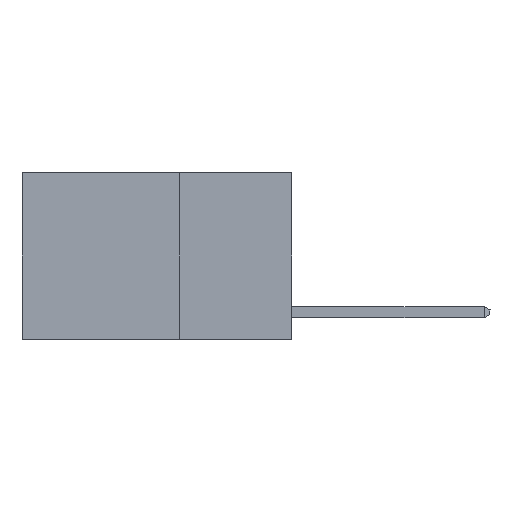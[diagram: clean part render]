
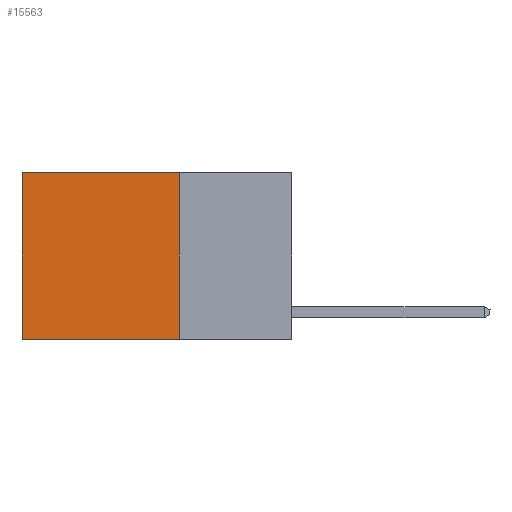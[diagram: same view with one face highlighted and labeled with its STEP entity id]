
A CAD part, left-side view. The second image highlights one B-rep face of the part: STEP entity #15563.
In plain terms, the highlighted planar face has unit normal (-1, 0, 0).
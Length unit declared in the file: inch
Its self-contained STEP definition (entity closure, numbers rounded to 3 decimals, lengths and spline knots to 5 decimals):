
#2061 = CARTESIAN_POINT ( 'NONE',  ( 0.2625, 0.25, -0.37 ) ) ;
#2104 = ORIENTED_EDGE ( 'NONE', *, *, #2161, .T. ) ;
#2161 = EDGE_CURVE ( 'NONE', #17631, #2592, #10800, .T. ) ;
#2592 = VERTEX_POINT ( 'NONE', #8706 ) ;
#2977 = CARTESIAN_POINT ( 'NONE',  ( 0.2625, 0.6, -0.37 ) ) ;
#3079 = CARTESIAN_POINT ( 'NONE',  ( 0.2625, 0.25, 0. ) ) ;
#4756 = ORIENTED_EDGE ( 'NONE', *, *, #24440, .F. ) ;
#4906 = CARTESIAN_POINT ( 'NONE',  ( 0.2625, 0.25, -0.37 ) ) ;
#5278 = FACE_OUTER_BOUND ( 'NONE', #20520, .T. ) ;
#6671 = ORIENTED_EDGE ( 'NONE', *, *, #13740, .F. ) ;
#7311 = VERTEX_POINT ( 'NONE', #2061 ) ;
#7392 = ORIENTED_EDGE ( 'NONE', *, *, #20738, .T. ) ;
#7588 = VECTOR ( 'NONE', #20068, 39.37008 ) ;
#8706 = CARTESIAN_POINT ( 'NONE',  ( 0.2625, 0.6, 0. ) ) ;
#8892 = DIRECTION ( 'NONE',  ( 0., 1., 0. ) ) ;
#8920 = CARTESIAN_POINT ( 'NONE',  ( 0.2625, 0.25, 0. ) ) ;
#9832 = CARTESIAN_POINT ( 'NONE',  ( 0.2625, 0.6, 0. ) ) ;
#9870 = DIRECTION ( 'NONE',  ( 0., 1., 0. ) ) ;
#9980 = LINE ( 'NONE', #9832, #12978 ) ;
#10800 = LINE ( 'NONE', #22239, #25747 ) ;
#11421 = AXIS2_PLACEMENT_3D ( 'NONE', #3079, #18039, #12015 ) ;
#12002 = VERTEX_POINT ( 'NONE', #2977 ) ;
#12015 = DIRECTION ( 'NONE',  ( 0., 0., -1. ) ) ;
#12978 = VECTOR ( 'NONE', #18632, 39.37008 ) ;
#13740 = EDGE_CURVE ( 'NONE', #17631, #7311, #26659, .T. ) ;
#13989 = LINE ( 'NONE', #4906, #19215 ) ;
#15563 = ADVANCED_FACE ( 'NONE', ( #5278 ), #23154, .F. ) ;
#17631 = VERTEX_POINT ( 'NONE', #25303 ) ;
#18039 = DIRECTION ( 'NONE',  ( 1., 0., 0. ) ) ;
#18632 = DIRECTION ( 'NONE',  ( 0., 0., -1. ) ) ;
#19215 = VECTOR ( 'NONE', #9870, 39.37008 ) ;
#20068 = DIRECTION ( 'NONE',  ( 0., 0., -1. ) ) ;
#20520 = EDGE_LOOP ( 'NONE', ( #7392, #4756, #6671, #2104 ) ) ;
#20738 = EDGE_CURVE ( 'NONE', #2592, #12002, #9980, .T. ) ;
#22239 = CARTESIAN_POINT ( 'NONE',  ( 0.2625, 0.25, 0. ) ) ;
#23154 = PLANE ( 'NONE',  #11421 ) ;
#24440 = EDGE_CURVE ( 'NONE', #7311, #12002, #13989, .T. ) ;
#25303 = CARTESIAN_POINT ( 'NONE',  ( 0.2625, 0.25, 0. ) ) ;
#25747 = VECTOR ( 'NONE', #8892, 39.37008 ) ;
#26659 = LINE ( 'NONE', #8920, #7588 ) ;
